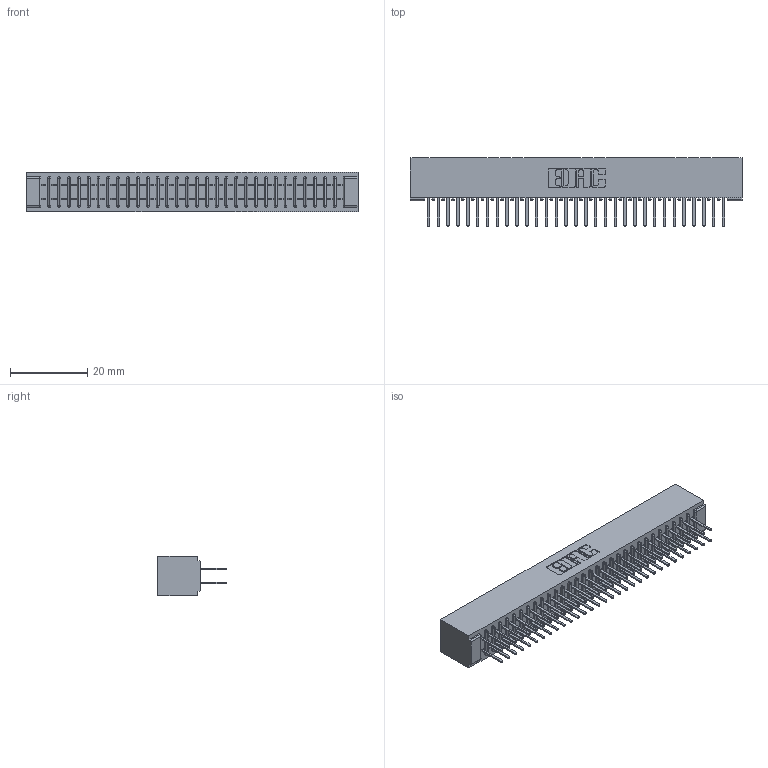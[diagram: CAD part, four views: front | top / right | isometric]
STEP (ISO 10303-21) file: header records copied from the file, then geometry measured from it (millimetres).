
FILE_DESCRIPTION (( 'STEP AP203' ), '1' );
FILE_NAME ('341-062-521-201.STEP', '2018-08-07T17:49:05', ( '' ), ( '' ), 'SwSTEP 2.0', 'SolidWorks 2016', '' );
FILE_SCHEMA (( 'CONFIG_CONTROL_DESIGN' ));
Length unit declared in the file: inch
Products named in the file (3): 341-062-521-201; 341 Part_No Mounting Lugs; 341-292-001_341-292-121
Assembly tree (63 placements, depth 2):
  341-062-521-201
    341 Part_No Mounting Lugs
    341-292-001_341-292-121  x62
Bounding box: 85.72 x 17.7 x 10.16 mm (x, y, z)
Volume: 6603.5 mm3; surface area: 12310.1 mm2
Topology: 63 solids, 63 shells, 4200 faces, 12165 edges, 7878 vertices
Faces by surface type: plane 2544, cylinder 1532, sphere 64, torus 60
Entity records: 38704 total; most frequent: CARTESIAN_POINT 6433, ORIENTED_EDGE 6390, DIRECTION 6249, EDGE_CURVE 3195, LINE 2573, VECTOR 2573, VERTEX_POINT 2022, AXIS2_PLACEMENT_3D 1838
